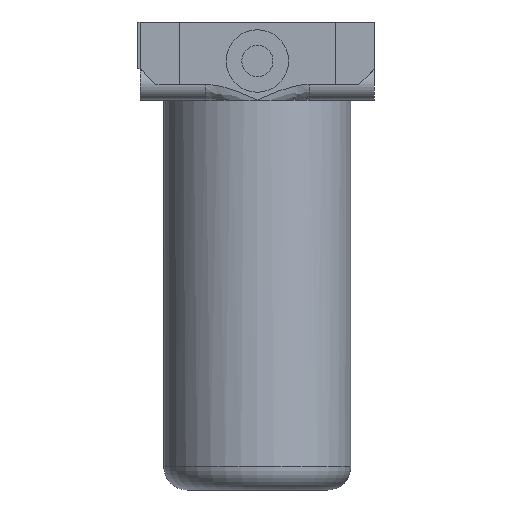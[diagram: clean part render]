
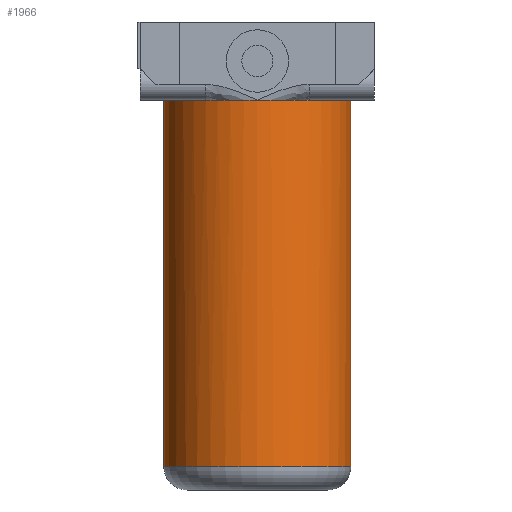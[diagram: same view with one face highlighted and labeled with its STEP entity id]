
A CAD part, front view. The second image highlights one B-rep face of the part: STEP entity #1966.
In plain terms, the highlighted cylindrical face has radius 15.24 mm (diameter 30.48 mm), a partial arc.
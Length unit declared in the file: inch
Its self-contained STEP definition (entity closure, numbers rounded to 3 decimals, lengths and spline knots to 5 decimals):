
#73 = CIRCLE ( 'NONE', #2260, 0.6 ) ;
#78 = CARTESIAN_POINT ( 'NONE',  ( 0., 0., 2.5 ) ) ;
#100 = FACE_OUTER_BOUND ( 'NONE', #703, .T. ) ;
#113 = CARTESIAN_POINT ( 'NONE',  ( 0.6, 0., 2.5 ) ) ;
#135 = DIRECTION ( 'NONE',  ( 0., 0., -1. ) ) ;
#225 = DIRECTION ( 'NONE',  ( 1., 0., 0. ) ) ;
#229 = ORIENTED_EDGE ( 'NONE', *, *, #1718, .F. ) ;
#263 = CARTESIAN_POINT ( 'NONE',  ( -0.6, 0., 2.5 ) ) ;
#281 = ORIENTED_EDGE ( 'NONE', *, *, #1588, .T. ) ;
#319 = VERTEX_POINT ( 'NONE', #263 ) ;
#334 = EDGE_CURVE ( 'NONE', #957, #1906, #1717, .T. ) ;
#437 = DIRECTION ( 'NONE',  ( 0., 0., 1. ) ) ;
#498 = VERTEX_POINT ( 'NONE', #1967 ) ;
#559 = CIRCLE ( 'NONE', #706, 0.6 ) ;
#614 = CARTESIAN_POINT ( 'NONE',  ( 0., 0., 0.15 ) ) ;
#643 = EDGE_CURVE ( 'NONE', #319, #1655, #1245, .T. ) ;
#664 = AXIS2_PLACEMENT_3D ( 'NONE', #614, #1259, #1863 ) ;
#696 = DIRECTION ( 'NONE',  ( 0., 0., 1. ) ) ;
#703 = EDGE_LOOP ( 'NONE', ( #229, #1577, #1708, #893, #1165, #822, #281 ) ) ;
#706 = AXIS2_PLACEMENT_3D ( 'NONE', #1430, #2036, #1820 ) ;
#728 = DIRECTION ( 'NONE',  ( 0., 0., 1. ) ) ;
#791 = EDGE_CURVE ( 'NONE', #1890, #957, #559, .T. ) ;
#822 = ORIENTED_EDGE ( 'NONE', *, *, #643, .T. ) ;
#886 = VECTOR ( 'NONE', #1400, 39.37008 ) ;
#893 = ORIENTED_EDGE ( 'NONE', *, *, #1873, .F. ) ;
#921 = CARTESIAN_POINT ( 'NONE',  ( 0., -0.6, 2.5 ) ) ;
#957 = VERTEX_POINT ( 'NONE', #1055 ) ;
#1022 = CARTESIAN_POINT ( 'NONE',  ( -0.6, 0., 0.15 ) ) ;
#1055 = CARTESIAN_POINT ( 'NONE',  ( 0.33166, -0.5, 2.5 ) ) ;
#1156 = CARTESIAN_POINT ( 'NONE',  ( 0., 0., 2.5 ) ) ;
#1165 = ORIENTED_EDGE ( 'NONE', *, *, #1916, .F. ) ;
#1194 = LINE ( 'NONE', #2303, #2217 ) ;
#1245 = LINE ( 'NONE', #1585, #886 ) ;
#1259 = DIRECTION ( 'NONE',  ( 0., 0., 1. ) ) ;
#1323 = CARTESIAN_POINT ( 'NONE',  ( 0., 0., 2.5 ) ) ;
#1400 = DIRECTION ( 'NONE',  ( 0., 0., -1. ) ) ;
#1430 = CARTESIAN_POINT ( 'NONE',  ( 0., 0., 2.5 ) ) ;
#1463 = AXIS2_PLACEMENT_3D ( 'NONE', #1865, #437, #225 ) ;
#1520 = DIRECTION ( 'NONE',  ( 1., 0., 0. ) ) ;
#1541 = AXIS2_PLACEMENT_3D ( 'NONE', #1156, #135, #1777 ) ;
#1577 = ORIENTED_EDGE ( 'NONE', *, *, #334, .F. ) ;
#1585 = CARTESIAN_POINT ( 'NONE',  ( -0.6, 0., 2.5 ) ) ;
#1588 = EDGE_CURVE ( 'NONE', #1655, #498, #2330, .T. ) ;
#1655 = VERTEX_POINT ( 'NONE', #1022 ) ;
#1685 = CYLINDRICAL_SURFACE ( 'NONE', #1541, 0.6 ) ;
#1708 = ORIENTED_EDGE ( 'NONE', *, *, #791, .F. ) ;
#1709 = CIRCLE ( 'NONE', #2194, 0.6 ) ;
#1717 = CIRCLE ( 'NONE', #1463, 0.6 ) ;
#1718 = EDGE_CURVE ( 'NONE', #1906, #498, #1194, .T. ) ;
#1777 = DIRECTION ( 'NONE',  ( -1., 0., 0. ) ) ;
#1786 = VERTEX_POINT ( 'NONE', #2529 ) ;
#1820 = DIRECTION ( 'NONE',  ( 1., 0., 0. ) ) ;
#1863 = DIRECTION ( 'NONE',  ( 1., 0., 0. ) ) ;
#1865 = CARTESIAN_POINT ( 'NONE',  ( 0., 0., 2.5 ) ) ;
#1873 = EDGE_CURVE ( 'NONE', #1786, #1890, #73, .T. ) ;
#1890 = VERTEX_POINT ( 'NONE', #921 ) ;
#1891 = DIRECTION ( 'NONE',  ( 0., 0., -1. ) ) ;
#1906 = VERTEX_POINT ( 'NONE', #113 ) ;
#1916 = EDGE_CURVE ( 'NONE', #319, #1786, #1709, .T. ) ;
#1966 = ADVANCED_FACE ( 'NONE', ( #100 ), #1685, .T. ) ;
#1967 = CARTESIAN_POINT ( 'NONE',  ( 0.6, 0., 0.15 ) ) ;
#2036 = DIRECTION ( 'NONE',  ( 0., 0., 1. ) ) ;
#2194 = AXIS2_PLACEMENT_3D ( 'NONE', #78, #696, #2341 ) ;
#2217 = VECTOR ( 'NONE', #1891, 39.37008 ) ;
#2260 = AXIS2_PLACEMENT_3D ( 'NONE', #1323, #728, #1520 ) ;
#2303 = CARTESIAN_POINT ( 'NONE',  ( 0.6, 0., 2.5 ) ) ;
#2330 = CIRCLE ( 'NONE', #664, 0.6 ) ;
#2341 = DIRECTION ( 'NONE',  ( 1., 0., 0. ) ) ;
#2529 = CARTESIAN_POINT ( 'NONE',  ( -0.33166, -0.5, 2.5 ) ) ;
